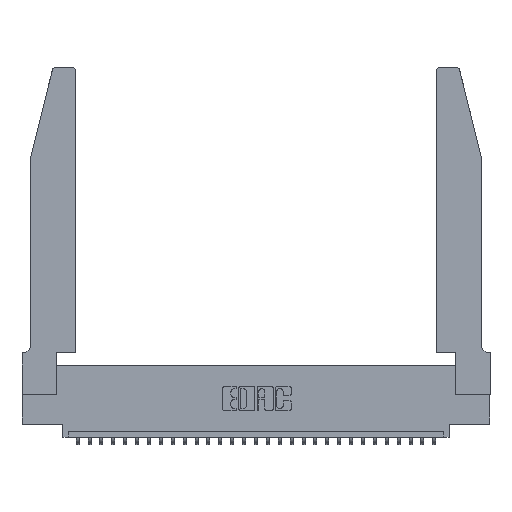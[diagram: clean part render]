
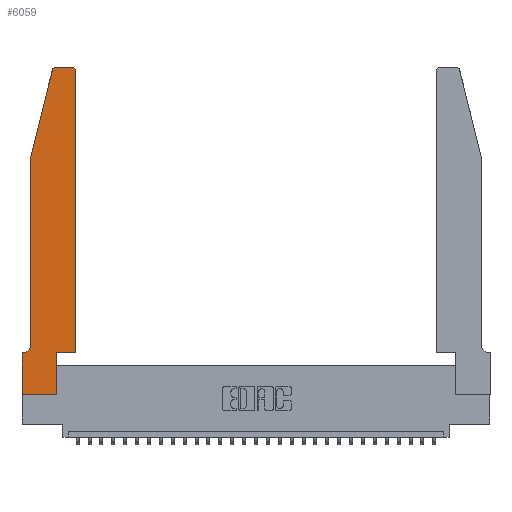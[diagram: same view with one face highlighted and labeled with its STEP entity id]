
A CAD part, top view. The second image highlights one B-rep face of the part: STEP entity #6059.
In plain terms, the highlighted planar face has unit normal (0, 0, 1).
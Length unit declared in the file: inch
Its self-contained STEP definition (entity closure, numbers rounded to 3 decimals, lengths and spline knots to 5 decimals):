
#92 = CARTESIAN_POINT ( 'NONE',  ( 0.0755, 2., 0.37 ) ) ;
#394 = EDGE_CURVE ( 'NONE', #534, #5634, #26644, .T. ) ;
#534 = VERTEX_POINT ( 'NONE', #19026 ) ;
#682 = CARTESIAN_POINT ( 'NONE',  ( 0.4505, 0.35, 0.37 ) ) ;
#1310 = EDGE_CURVE ( 'NONE', #5634, #6117, #9691, .T. ) ;
#1700 = ORIENTED_EDGE ( 'NONE', *, *, #29458, .T. ) ;
#1832 = LINE ( 'NONE', #26630, #16642 ) ;
#2055 = LINE ( 'NONE', #22056, #21824 ) ;
#2351 = AXIS2_PLACEMENT_3D ( 'NONE', #15555, #20250, #13010 ) ;
#2373 = ORIENTED_EDGE ( 'NONE', *, *, #12106, .T. ) ;
#2697 = EDGE_CURVE ( 'NONE', #16098, #24398, #11640, .T. ) ;
#2769 = VECTOR ( 'NONE', #10805, 39.37008 ) ;
#3285 = VERTEX_POINT ( 'NONE', #9960 ) ;
#3548 = VECTOR ( 'NONE', #20501, 39.37008 ) ;
#3871 = ORIENTED_EDGE ( 'NONE', *, *, #12321, .T. ) ;
#4164 = CARTESIAN_POINT ( 'NONE',  ( 0.284, 2.72, 0.37 ) ) ;
#4440 = EDGE_CURVE ( 'NONE', #3285, #15216, #1832, .T. ) ;
#5187 = ORIENTED_EDGE ( 'NONE', *, *, #1310, .T. ) ;
#5498 = AXIS2_PLACEMENT_3D ( 'NONE', #15122, #5934, #17470 ) ;
#5634 = VERTEX_POINT ( 'NONE', #27294 ) ;
#5934 = DIRECTION ( 'NONE',  ( 0., 0., 1. ) ) ;
#6059 = ADVANCED_FACE ( 'NONE', ( #25077 ), #28869, .T. ) ;
#6117 = VERTEX_POINT ( 'NONE', #13399 ) ;
#6261 = DIRECTION ( 'NONE',  ( 0., 0., 1. ) ) ;
#6743 = CARTESIAN_POINT ( 'NONE',  ( 0.2865, 0.35, 0.37 ) ) ;
#7021 = CARTESIAN_POINT ( 'NONE',  ( 0.0055, 0.35, 0.37 ) ) ;
#7480 = VERTEX_POINT ( 'NONE', #12475 ) ;
#8791 = DIRECTION ( 'NONE',  ( 1., 0., 0. ) ) ;
#9418 = CIRCLE ( 'NONE', #22302, 0.03 ) ;
#9553 = DIRECTION ( 'NONE',  ( 0., 0., 1. ) ) ;
#9691 = LINE ( 'NONE', #27544, #3548 ) ;
#9754 = ORIENTED_EDGE ( 'NONE', *, *, #9779, .T. ) ;
#9779 = EDGE_CURVE ( 'NONE', #17462, #10337, #2055, .T. ) ;
#9786 = CARTESIAN_POINT ( 'NONE',  ( 0.4505, 2.72, 0.37 ) ) ;
#9960 = CARTESIAN_POINT ( 'NONE',  ( 0., 0., 0.37 ) ) ;
#10337 = VERTEX_POINT ( 'NONE', #9786 ) ;
#10401 = DIRECTION ( 'NONE',  ( 0., 1., 0. ) ) ;
#10805 = DIRECTION ( 'NONE',  ( -1., 0., 0. ) ) ;
#11282 = CARTESIAN_POINT ( 'NONE',  ( 0., 0., 0.37 ) ) ;
#11492 = DIRECTION ( 'NONE',  ( 0., 1., 0. ) ) ;
#11496 = CIRCLE ( 'NONE', #23407, 0.03 ) ;
#11622 = ORIENTED_EDGE ( 'NONE', *, *, #14977, .T. ) ;
#11640 = LINE ( 'NONE', #24198, #18525 ) ;
#11912 = ORIENTED_EDGE ( 'NONE', *, *, #21244, .T. ) ;
#12106 = EDGE_CURVE ( 'NONE', #6117, #16589, #23895, .T. ) ;
#12261 = VECTOR ( 'NONE', #19738, 39.37008 ) ;
#12321 = EDGE_CURVE ( 'NONE', #7480, #3285, #15616, .T. ) ;
#12475 = CARTESIAN_POINT ( 'NONE',  ( 0., 0.35, 0.37 ) ) ;
#12878 = DIRECTION ( 'NONE',  ( 1., 0., 0. ) ) ;
#13010 = DIRECTION ( 'NONE',  ( -1., 0., 0. ) ) ;
#13037 = CARTESIAN_POINT ( 'NONE',  ( 0.0755, 0.35, 0.37 ) ) ;
#13399 = CARTESIAN_POINT ( 'NONE',  ( 0.0755, 0.42, 0.37 ) ) ;
#14452 = VECTOR ( 'NONE', #25314, 39.37008 ) ;
#14618 = CARTESIAN_POINT ( 'NONE',  ( 0.4205, 2.75, 0.37 ) ) ;
#14977 = EDGE_CURVE ( 'NONE', #16589, #7480, #16150, .T. ) ;
#15122 = CARTESIAN_POINT ( 'NONE',  ( 0., 0.35, 0.37 ) ) ;
#15216 = VERTEX_POINT ( 'NONE', #25473 ) ;
#15292 = VECTOR ( 'NONE', #11492, 39.37008 ) ;
#15555 = CARTESIAN_POINT ( 'NONE',  ( 0.0055, 0.42, 0.37 ) ) ;
#15616 = LINE ( 'NONE', #11282, #19230 ) ;
#16098 = VERTEX_POINT ( 'NONE', #14618 ) ;
#16150 = LINE ( 'NONE', #13037, #2769 ) ;
#16589 = VERTEX_POINT ( 'NONE', #7021 ) ;
#16642 = VECTOR ( 'NONE', #12878, 39.37008 ) ;
#17462 = VERTEX_POINT ( 'NONE', #682 ) ;
#17470 = DIRECTION ( 'NONE',  ( 1., 0., 0. ) ) ;
#18238 = CARTESIAN_POINT ( 'NONE',  ( 0.2865, 0.35, 0.37 ) ) ;
#18525 = VECTOR ( 'NONE', #21976, 39.37008 ) ;
#18919 = ORIENTED_EDGE ( 'NONE', *, *, #394, .T. ) ;
#19026 = CARTESIAN_POINT ( 'NONE',  ( 0.25487, 2.72718, 0.37 ) ) ;
#19230 = VECTOR ( 'NONE', #29687, 39.37008 ) ;
#19738 = DIRECTION ( 'NONE',  ( 1., 0., 0. ) ) ;
#20250 = DIRECTION ( 'NONE',  ( 0., 0., -1. ) ) ;
#20310 = EDGE_LOOP ( 'NONE', ( #21505, #1700, #18919, #5187, #2373, #11622, #3871, #25625, #27880, #22280, #9754, #11912 ) ) ;
#20501 = DIRECTION ( 'NONE',  ( 0., -1., 0. ) ) ;
#21244 = EDGE_CURVE ( 'NONE', #10337, #16098, #9418, .T. ) ;
#21308 = CARTESIAN_POINT ( 'NONE',  ( 0.4205, 2.72, 0.37 ) ) ;
#21505 = ORIENTED_EDGE ( 'NONE', *, *, #2697, .T. ) ;
#21824 = VECTOR ( 'NONE', #10401, 39.37008 ) ;
#21952 = LINE ( 'NONE', #26648, #12261 ) ;
#21976 = DIRECTION ( 'NONE',  ( -1., 0., 0. ) ) ;
#22056 = CARTESIAN_POINT ( 'NONE',  ( 0.4505, 0.35, 0.37 ) ) ;
#22280 = ORIENTED_EDGE ( 'NONE', *, *, #27271, .T. ) ;
#22302 = AXIS2_PLACEMENT_3D ( 'NONE', #21308, #9553, #23625 ) ;
#23407 = AXIS2_PLACEMENT_3D ( 'NONE', #4164, #6261, #8791 ) ;
#23625 = DIRECTION ( 'NONE',  ( 1., 0., 0. ) ) ;
#23875 = VERTEX_POINT ( 'NONE', #18238 ) ;
#23895 = CIRCLE ( 'NONE', #2351, 0.07 ) ;
#24198 = CARTESIAN_POINT ( 'NONE',  ( 0.2605, 2.75, 0.37 ) ) ;
#24398 = VERTEX_POINT ( 'NONE', #24474 ) ;
#24474 = CARTESIAN_POINT ( 'NONE',  ( 0.284, 2.75, 0.37 ) ) ;
#25062 = EDGE_CURVE ( 'NONE', #15216, #23875, #28565, .T. ) ;
#25077 = FACE_OUTER_BOUND ( 'NONE', #20310, .T. ) ;
#25314 = DIRECTION ( 'NONE',  ( -0.239, -0.971, 0. ) ) ;
#25473 = CARTESIAN_POINT ( 'NONE',  ( 0.2865, 0., 0.37 ) ) ;
#25625 = ORIENTED_EDGE ( 'NONE', *, *, #4440, .T. ) ;
#26630 = CARTESIAN_POINT ( 'NONE',  ( 0., 0., 0.37 ) ) ;
#26644 = LINE ( 'NONE', #92, #14452 ) ;
#26648 = CARTESIAN_POINT ( 'NONE',  ( 0.4505, 0.35, 0.37 ) ) ;
#27271 = EDGE_CURVE ( 'NONE', #23875, #17462, #21952, .T. ) ;
#27294 = CARTESIAN_POINT ( 'NONE',  ( 0.0755, 2., 0.37 ) ) ;
#27544 = CARTESIAN_POINT ( 'NONE',  ( 0.0755, 2., 0.37 ) ) ;
#27880 = ORIENTED_EDGE ( 'NONE', *, *, #25062, .T. ) ;
#28565 = LINE ( 'NONE', #6743, #15292 ) ;
#28869 = PLANE ( 'NONE',  #5498 ) ;
#29458 = EDGE_CURVE ( 'NONE', #24398, #534, #11496, .T. ) ;
#29687 = DIRECTION ( 'NONE',  ( 0., -1., 0. ) ) ;
